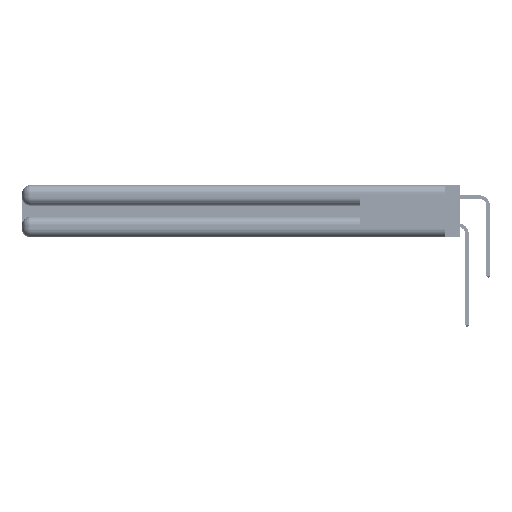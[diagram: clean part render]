
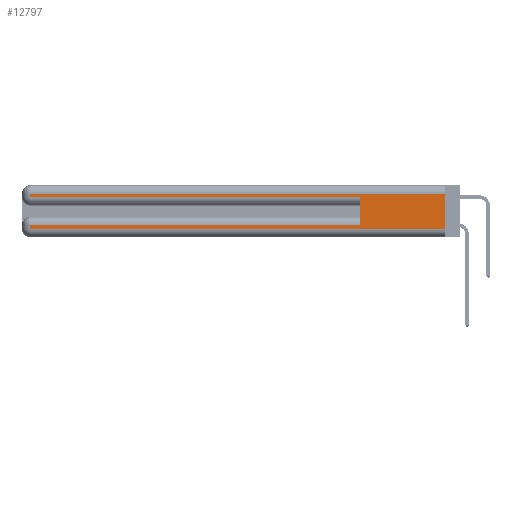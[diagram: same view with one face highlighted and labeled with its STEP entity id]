
A CAD part, left-side view. The second image highlights one B-rep face of the part: STEP entity #12797.
In plain terms, the highlighted planar face has unit normal (-1, 0, 0).
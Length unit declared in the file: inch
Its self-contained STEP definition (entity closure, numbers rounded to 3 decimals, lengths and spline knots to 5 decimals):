
#4395 = DIRECTION ( 'NONE',  ( 0., -1., 0. ) ) ;
#4489 = CARTESIAN_POINT ( 'NONE',  ( 0., 2.94, 0.31 ) ) ;
#5545 = VERTEX_POINT ( 'NONE', #51975 ) ;
#6849 = CARTESIAN_POINT ( 'NONE',  ( 0., 0., 0.31 ) ) ;
#9474 = PLANE ( 'NONE',  #53108 ) ;
#10196 = VERTEX_POINT ( 'NONE', #20134 ) ;
#11592 = VECTOR ( 'NONE', #4395, 39.37008 ) ;
#11622 = LINE ( 'NONE', #24133, #56542 ) ;
#12797 = ADVANCED_FACE ( 'NONE', ( #50810 ), #9474, .F. ) ;
#13053 = EDGE_CURVE ( 'NONE', #53621, #15122, #15614, .T. ) ;
#14375 = VECTOR ( 'NONE', #32801, 39.37008 ) ;
#15122 = VERTEX_POINT ( 'NONE', #44433 ) ;
#15502 = VECTOR ( 'NONE', #56087, 39.37008 ) ;
#15614 = LINE ( 'NONE', #38188, #50088 ) ;
#15736 = DIRECTION ( 'NONE',  ( 0., 0., -1. ) ) ;
#16851 = DIRECTION ( 'NONE',  ( 0., 1., 0. ) ) ;
#18562 = CARTESIAN_POINT ( 'NONE',  ( 0., 0., 0.37 ) ) ;
#18800 = VERTEX_POINT ( 'NONE', #58024 ) ;
#19102 = VECTOR ( 'NONE', #36030, 39.37008 ) ;
#20134 = CARTESIAN_POINT ( 'NONE',  ( 0., 0., 0.31 ) ) ;
#21555 = CARTESIAN_POINT ( 'NONE',  ( 0., 0.6, 0.285 ) ) ;
#21822 = ORIENTED_EDGE ( 'NONE', *, *, #13053, .T. ) ;
#22825 = CARTESIAN_POINT ( 'NONE',  ( 0., 0.6, 0.145 ) ) ;
#23073 = DIRECTION ( 'NONE',  ( 0., 0., -1. ) ) ;
#23209 = DIRECTION ( 'NONE',  ( 0., 0., 1. ) ) ;
#24133 = CARTESIAN_POINT ( 'NONE',  ( 0., 0., 0.285 ) ) ;
#24675 = ORIENTED_EDGE ( 'NONE', *, *, #45022, .T. ) ;
#26433 = VECTOR ( 'NONE', #16851, 39.37008 ) ;
#28917 = ORIENTED_EDGE ( 'NONE', *, *, #58089, .T. ) ;
#32801 = DIRECTION ( 'NONE',  ( 0., 0., -1. ) ) ;
#33264 = EDGE_LOOP ( 'NONE', ( #47681, #39341, #21822, #55912, #33606, #53240, #24675, #28917 ) ) ;
#33606 = ORIENTED_EDGE ( 'NONE', *, *, #42432, .F. ) ;
#33903 = LINE ( 'NONE', #49326, #19102 ) ;
#35319 = EDGE_CURVE ( 'NONE', #15122, #45666, #11622, .T. ) ;
#36030 = DIRECTION ( 'NONE',  ( 0., 0., -1. ) ) ;
#37625 = EDGE_CURVE ( 'NONE', #10196, #5545, #33903, .T. ) ;
#37963 = EDGE_CURVE ( 'NONE', #10196, #53621, #38056, .T. ) ;
#38056 = LINE ( 'NONE', #6849, #15502 ) ;
#38188 = CARTESIAN_POINT ( 'NONE',  ( 0., 2.94, 0.37 ) ) ;
#39273 = CARTESIAN_POINT ( 'NONE',  ( 0., 0., 0.085 ) ) ;
#39341 = ORIENTED_EDGE ( 'NONE', *, *, #37963, .T. ) ;
#40380 = CARTESIAN_POINT ( 'NONE',  ( 0., 0., 0.06 ) ) ;
#42432 = EDGE_CURVE ( 'NONE', #54890, #45666, #46395, .T. ) ;
#44433 = CARTESIAN_POINT ( 'NONE',  ( 0., 2.94, 0.285 ) ) ;
#44661 = EDGE_CURVE ( 'NONE', #54890, #56305, #57965, .T. ) ;
#45022 = EDGE_CURVE ( 'NONE', #56305, #18800, #50258, .T. ) ;
#45666 = VERTEX_POINT ( 'NONE', #21555 ) ;
#46395 = LINE ( 'NONE', #22825, #56824 ) ;
#47681 = ORIENTED_EDGE ( 'NONE', *, *, #37625, .F. ) ;
#49326 = CARTESIAN_POINT ( 'NONE',  ( 0., 0., 0.37 ) ) ;
#49976 = DIRECTION ( 'NONE',  ( 1., 0., 0. ) ) ;
#50088 = VECTOR ( 'NONE', #15736, 39.37008 ) ;
#50258 = LINE ( 'NONE', #55064, #14375 ) ;
#50810 = FACE_OUTER_BOUND ( 'NONE', #33264, .T. ) ;
#51017 = DIRECTION ( 'NONE',  ( 0., -1., 0. ) ) ;
#51552 = CARTESIAN_POINT ( 'NONE',  ( 0., 2.94, 0.085 ) ) ;
#51975 = CARTESIAN_POINT ( 'NONE',  ( 0., 0., 0.06 ) ) ;
#53108 = AXIS2_PLACEMENT_3D ( 'NONE', #18562, #49976, #23073 ) ;
#53240 = ORIENTED_EDGE ( 'NONE', *, *, #44661, .T. ) ;
#53621 = VERTEX_POINT ( 'NONE', #4489 ) ;
#54013 = CARTESIAN_POINT ( 'NONE',  ( 0., 0.6, 0.085 ) ) ;
#54890 = VERTEX_POINT ( 'NONE', #54013 ) ;
#55064 = CARTESIAN_POINT ( 'NONE',  ( 0., 2.94, 0.37 ) ) ;
#55912 = ORIENTED_EDGE ( 'NONE', *, *, #35319, .T. ) ;
#56087 = DIRECTION ( 'NONE',  ( 0., 1., 0. ) ) ;
#56305 = VERTEX_POINT ( 'NONE', #51552 ) ;
#56542 = VECTOR ( 'NONE', #51017, 39.37008 ) ;
#56824 = VECTOR ( 'NONE', #23209, 39.37008 ) ;
#57919 = LINE ( 'NONE', #40380, #11592 ) ;
#57965 = LINE ( 'NONE', #39273, #26433 ) ;
#58024 = CARTESIAN_POINT ( 'NONE',  ( 0., 2.94, 0.06 ) ) ;
#58089 = EDGE_CURVE ( 'NONE', #18800, #5545, #57919, .T. ) ;
